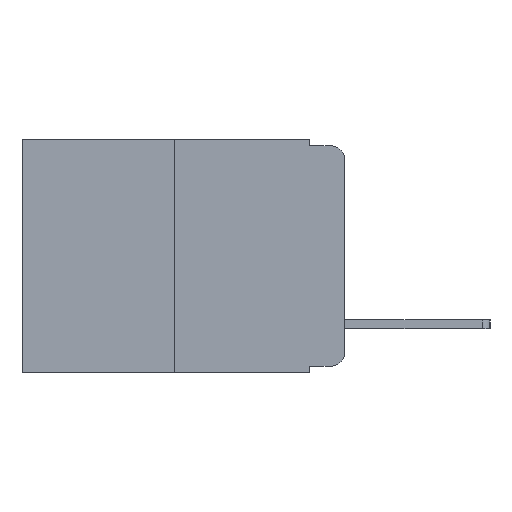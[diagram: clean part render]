
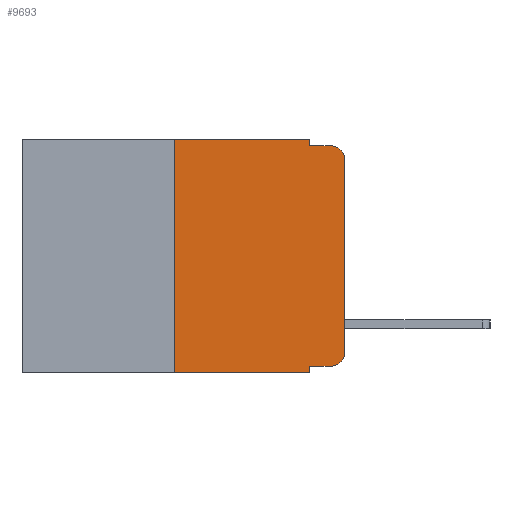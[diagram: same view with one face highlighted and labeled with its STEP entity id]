
A CAD part, left-side view. The second image highlights one B-rep face of the part: STEP entity #9693.
In plain terms, the highlighted planar face has unit normal (-1, 0, 0).
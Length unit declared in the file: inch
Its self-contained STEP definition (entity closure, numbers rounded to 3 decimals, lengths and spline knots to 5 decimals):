
#30 = VERTEX_POINT ( 'NONE', #16973 ) ;
#135 = DIRECTION ( 'NONE',  ( 0., 0., -1. ) ) ;
#195 = DIRECTION ( 'NONE',  ( -1., 0., 0. ) ) ;
#209 = EDGE_CURVE ( 'NONE', #7484, #30, #6222, .T. ) ;
#462 = DIRECTION ( 'NONE',  ( 0., 0., -1. ) ) ;
#816 = AXIS2_PLACEMENT_3D ( 'NONE', #6064, #195, #16613 ) ;
#1087 = EDGE_CURVE ( 'NONE', #3175, #30, #12087, .T. ) ;
#1173 = DIRECTION ( 'NONE',  ( -1., 0., 0. ) ) ;
#1286 = VERTEX_POINT ( 'NONE', #18351 ) ;
#1364 = EDGE_CURVE ( 'NONE', #14640, #9754, #12325, .T. ) ;
#1524 = CARTESIAN_POINT ( 'NONE',  ( 0., 0.25, -0.343 ) ) ;
#2122 = CARTESIAN_POINT ( 'NONE',  ( 0., 0.473, 0. ) ) ;
#2200 = LINE ( 'NONE', #12823, #9278 ) ;
#2234 = EDGE_CURVE ( 'NONE', #11805, #3175, #2350, .T. ) ;
#2350 = LINE ( 'NONE', #14690, #9397 ) ;
#2797 = AXIS2_PLACEMENT_3D ( 'NONE', #2122, #9675, #462 ) ;
#2861 = VECTOR ( 'NONE', #12891, 39.37008 ) ;
#3175 = VERTEX_POINT ( 'NONE', #9562 ) ;
#3413 = ORIENTED_EDGE ( 'NONE', *, *, #15246, .T. ) ;
#3458 = CIRCLE ( 'NONE', #7127, 0.02 ) ;
#3528 = CARTESIAN_POINT ( 'NONE',  ( 0., 0.051, 0. ) ) ;
#4097 = VECTOR ( 'NONE', #135, 39.37008 ) ;
#4118 = ORIENTED_EDGE ( 'NONE', *, *, #17094, .F. ) ;
#4119 = FACE_OUTER_BOUND ( 'NONE', #4226, .T. ) ;
#4226 = EDGE_LOOP ( 'NONE', ( #8151, #17921, #15870, #11460, #5078, #13031, #4342, #4118, #9890, #3413 ) ) ;
#4342 = ORIENTED_EDGE ( 'NONE', *, *, #15138, .T. ) ;
#4589 = VERTEX_POINT ( 'NONE', #4891 ) ;
#4600 = CARTESIAN_POINT ( 'NONE',  ( 0., 0.25, 0. ) ) ;
#4646 = DIRECTION ( 'NONE',  ( 0., 0., 1. ) ) ;
#4891 = CARTESIAN_POINT ( 'NONE',  ( 0., 0.051, -0.343 ) ) ;
#5078 = ORIENTED_EDGE ( 'NONE', *, *, #1364, .F. ) ;
#5152 = VECTOR ( 'NONE', #12970, 39.37008 ) ;
#5754 = VECTOR ( 'NONE', #17723, 39.37008 ) ;
#6064 = CARTESIAN_POINT ( 'NONE',  ( 0., 0.02, -0.03 ) ) ;
#6218 = CARTESIAN_POINT ( 'NONE',  ( 0., 0.051, -0.333 ) ) ;
#6222 = LINE ( 'NONE', #11955, #5754 ) ;
#6838 = LINE ( 'NONE', #11499, #2861 ) ;
#7127 = AXIS2_PLACEMENT_3D ( 'NONE', #10226, #1173, #11670 ) ;
#7484 = VERTEX_POINT ( 'NONE', #13243 ) ;
#8072 = VECTOR ( 'NONE', #16213, 39.37008 ) ;
#8151 = ORIENTED_EDGE ( 'NONE', *, *, #2234, .T. ) ;
#8227 = PLANE ( 'NONE',  #2797 ) ;
#8793 = VECTOR ( 'NONE', #16176, 39.37008 ) ;
#8916 = CARTESIAN_POINT ( 'NONE',  ( 0., 0., -0.313 ) ) ;
#9049 = VERTEX_POINT ( 'NONE', #18168 ) ;
#9162 = LINE ( 'NONE', #17120, #5152 ) ;
#9278 = VECTOR ( 'NONE', #14218, 39.37008 ) ;
#9397 = VECTOR ( 'NONE', #4646, 39.37008 ) ;
#9562 = CARTESIAN_POINT ( 'NONE',  ( 0., 0., -0.03 ) ) ;
#9675 = DIRECTION ( 'NONE',  ( 1., 0., 0. ) ) ;
#9693 = ADVANCED_FACE ( 'NONE', ( #4119 ), #8227, .F. ) ;
#9754 = VERTEX_POINT ( 'NONE', #11221 ) ;
#9871 = CARTESIAN_POINT ( 'NONE',  ( 0., 0.473, 0. ) ) ;
#9890 = ORIENTED_EDGE ( 'NONE', *, *, #16181, .T. ) ;
#10226 = CARTESIAN_POINT ( 'NONE',  ( 0., 0.02, -0.313 ) ) ;
#11221 = CARTESIAN_POINT ( 'NONE',  ( 0., 0.051, 0. ) ) ;
#11460 = ORIENTED_EDGE ( 'NONE', *, *, #18002, .F. ) ;
#11499 = CARTESIAN_POINT ( 'NONE',  ( 0., 0.051, 0. ) ) ;
#11670 = DIRECTION ( 'NONE',  ( 0., 0., -1. ) ) ;
#11805 = VERTEX_POINT ( 'NONE', #8916 ) ;
#11852 = LINE ( 'NONE', #3528, #4097 ) ;
#11955 = CARTESIAN_POINT ( 'NONE',  ( 0., 0.051, -0.01 ) ) ;
#12087 = CIRCLE ( 'NONE', #816, 0.02 ) ;
#12325 = LINE ( 'NONE', #9871, #8072 ) ;
#12823 = CARTESIAN_POINT ( 'NONE',  ( 0., 0.473, -0.343 ) ) ;
#12891 = DIRECTION ( 'NONE',  ( 0., 0., -1. ) ) ;
#12970 = DIRECTION ( 'NONE',  ( 0., 0., 1. ) ) ;
#13031 = ORIENTED_EDGE ( 'NONE', *, *, #18901, .F. ) ;
#13243 = CARTESIAN_POINT ( 'NONE',  ( 0., 0.051, -0.01 ) ) ;
#14218 = DIRECTION ( 'NONE',  ( 0., -1., 0. ) ) ;
#14640 = VERTEX_POINT ( 'NONE', #4600 ) ;
#14690 = CARTESIAN_POINT ( 'NONE',  ( 0., 0., 0. ) ) ;
#15138 = EDGE_CURVE ( 'NONE', #16920, #4589, #2200, .T. ) ;
#15246 = EDGE_CURVE ( 'NONE', #9049, #11805, #3458, .T. ) ;
#15870 = ORIENTED_EDGE ( 'NONE', *, *, #209, .F. ) ;
#16176 = DIRECTION ( 'NONE',  ( 0., -1., 0. ) ) ;
#16181 = EDGE_CURVE ( 'NONE', #1286, #9049, #16206, .T. ) ;
#16206 = LINE ( 'NONE', #6218, #8793 ) ;
#16213 = DIRECTION ( 'NONE',  ( 0., -1., 0. ) ) ;
#16613 = DIRECTION ( 'NONE',  ( 0., 0., -1. ) ) ;
#16920 = VERTEX_POINT ( 'NONE', #1524 ) ;
#16973 = CARTESIAN_POINT ( 'NONE',  ( 0., 0.02, -0.01 ) ) ;
#17094 = EDGE_CURVE ( 'NONE', #1286, #4589, #11852, .T. ) ;
#17120 = CARTESIAN_POINT ( 'NONE',  ( 0., 0.25, 0. ) ) ;
#17723 = DIRECTION ( 'NONE',  ( 0., -1., 0. ) ) ;
#17921 = ORIENTED_EDGE ( 'NONE', *, *, #1087, .T. ) ;
#18002 = EDGE_CURVE ( 'NONE', #9754, #7484, #6838, .T. ) ;
#18168 = CARTESIAN_POINT ( 'NONE',  ( 0., 0.02, -0.333 ) ) ;
#18351 = CARTESIAN_POINT ( 'NONE',  ( 0., 0.051, -0.333 ) ) ;
#18901 = EDGE_CURVE ( 'NONE', #16920, #14640, #9162, .T. ) ;
